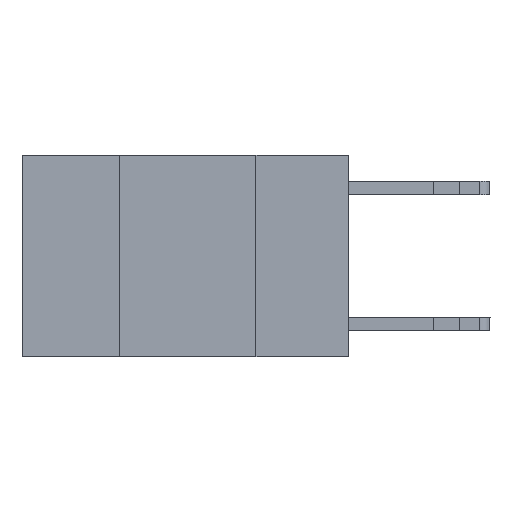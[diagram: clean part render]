
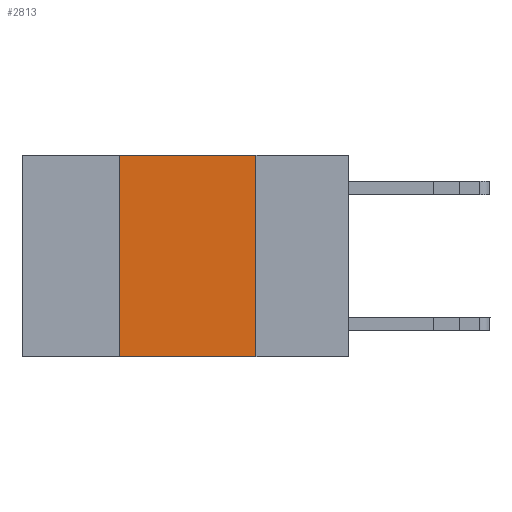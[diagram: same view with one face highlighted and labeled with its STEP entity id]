
A CAD part, left-side view. The second image highlights one B-rep face of the part: STEP entity #2813.
In plain terms, the highlighted planar face has unit normal (-1, 0, 0).
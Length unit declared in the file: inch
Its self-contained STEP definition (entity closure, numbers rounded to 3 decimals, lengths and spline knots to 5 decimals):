
#242 = VERTEX_POINT ( 'NONE', #9679 ) ;
#692 = VERTEX_POINT ( 'NONE', #7179 ) ;
#713 = DIRECTION ( 'NONE',  ( 0., 0., 1. ) ) ;
#765 = CARTESIAN_POINT ( 'NONE',  ( 0., 0.42, 0. ) ) ;
#1166 = VECTOR ( 'NONE', #10148, 39.37008 ) ;
#1951 = CARTESIAN_POINT ( 'NONE',  ( 0., 0.6, 0. ) ) ;
#1992 = CARTESIAN_POINT ( 'NONE',  ( 0., 0.42, 0. ) ) ;
#2813 = ADVANCED_FACE ( 'NONE', ( #4700 ), #5619, .F. ) ;
#2957 = DIRECTION ( 'NONE',  ( 0., -1., 0. ) ) ;
#3056 = LINE ( 'NONE', #11342, #10772 ) ;
#3078 = ORIENTED_EDGE ( 'NONE', *, *, #7291, .T. ) ;
#3250 = EDGE_LOOP ( 'NONE', ( #5566, #8891, #11200, #3078 ) ) ;
#3838 = EDGE_CURVE ( 'NONE', #692, #242, #3056, .T. ) ;
#4067 = EDGE_CURVE ( 'NONE', #11830, #692, #7075, .T. ) ;
#4487 = DIRECTION ( 'NONE',  ( 0., 0., -1. ) ) ;
#4610 = CARTESIAN_POINT ( 'NONE',  ( 0., 0.6, 0. ) ) ;
#4700 = FACE_OUTER_BOUND ( 'NONE', #3250, .T. ) ;
#5231 = VERTEX_POINT ( 'NONE', #10581 ) ;
#5566 = ORIENTED_EDGE ( 'NONE', *, *, #3838, .F. ) ;
#5619 = PLANE ( 'NONE',  #11777 ) ;
#6361 = LINE ( 'NONE', #11015, #8663 ) ;
#6557 = DIRECTION ( 'NONE',  ( 0., 0., -1. ) ) ;
#7075 = LINE ( 'NONE', #1951, #1166 ) ;
#7179 = CARTESIAN_POINT ( 'NONE',  ( 0., 0.17, 0. ) ) ;
#7291 = EDGE_CURVE ( 'NONE', #5231, #242, #6361, .T. ) ;
#7990 = LINE ( 'NONE', #765, #9968 ) ;
#8663 = VECTOR ( 'NONE', #2957, 39.37008 ) ;
#8891 = ORIENTED_EDGE ( 'NONE', *, *, #4067, .F. ) ;
#9485 = DIRECTION ( 'NONE',  ( 1., 0., 0. ) ) ;
#9679 = CARTESIAN_POINT ( 'NONE',  ( 0., 0.17, -0.37 ) ) ;
#9968 = VECTOR ( 'NONE', #713, 39.37008 ) ;
#10148 = DIRECTION ( 'NONE',  ( 0., -1., 0. ) ) ;
#10581 = CARTESIAN_POINT ( 'NONE',  ( 0., 0.42, -0.37 ) ) ;
#10740 = EDGE_CURVE ( 'NONE', #5231, #11830, #7990, .T. ) ;
#10772 = VECTOR ( 'NONE', #4487, 39.37008 ) ;
#11015 = CARTESIAN_POINT ( 'NONE',  ( 0., 0.6, -0.37 ) ) ;
#11200 = ORIENTED_EDGE ( 'NONE', *, *, #10740, .F. ) ;
#11342 = CARTESIAN_POINT ( 'NONE',  ( 0., 0.17, 0. ) ) ;
#11777 = AXIS2_PLACEMENT_3D ( 'NONE', #4610, #9485, #6557 ) ;
#11830 = VERTEX_POINT ( 'NONE', #1992 ) ;
